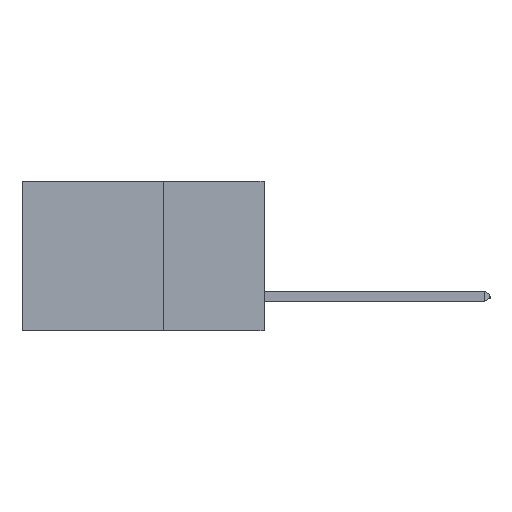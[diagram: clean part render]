
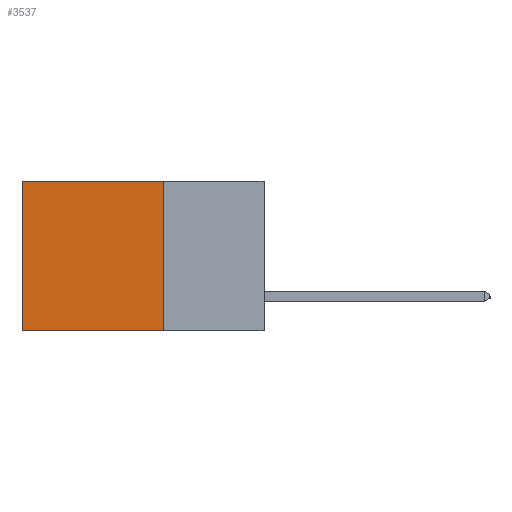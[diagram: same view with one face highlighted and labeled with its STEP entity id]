
A CAD part, left-side view. The second image highlights one B-rep face of the part: STEP entity #3537.
In plain terms, the highlighted planar face has unit normal (-1, 0, 0).
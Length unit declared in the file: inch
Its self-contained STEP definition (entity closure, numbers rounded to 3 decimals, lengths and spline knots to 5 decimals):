
#515 = VECTOR ( 'NONE', #7679, 39.37008 ) ;
#1892 = FACE_OUTER_BOUND ( 'NONE', #7209, .T. ) ;
#2263 = ORIENTED_EDGE ( 'NONE', *, *, #4184, .T. ) ;
#2540 = CARTESIAN_POINT ( 'NONE',  ( 0.298, 0.25, -0.37 ) ) ;
#2552 = CARTESIAN_POINT ( 'NONE',  ( 0.298, 0.25, -0.37 ) ) ;
#2980 = DIRECTION ( 'NONE',  ( 1., 0., 0. ) ) ;
#3294 = DIRECTION ( 'NONE',  ( 0., 0., -1. ) ) ;
#3537 = ADVANCED_FACE ( 'NONE', ( #1892 ), #13836, .F. ) ;
#3599 = VERTEX_POINT ( 'NONE', #7560 ) ;
#3607 = VECTOR ( 'NONE', #5527, 39.37008 ) ;
#4184 = EDGE_CURVE ( 'NONE', #3599, #9259, #11468, .T. ) ;
#4419 = LINE ( 'NONE', #2552, #515 ) ;
#4475 = ORIENTED_EDGE ( 'NONE', *, *, #8166, .F. ) ;
#5527 = DIRECTION ( 'NONE',  ( 0., 1., 0. ) ) ;
#7209 = EDGE_LOOP ( 'NONE', ( #2263, #10523, #4475, #12527 ) ) ;
#7462 = VECTOR ( 'NONE', #10243, 39.37008 ) ;
#7560 = CARTESIAN_POINT ( 'NONE',  ( 0.298, 0.6, 0. ) ) ;
#7679 = DIRECTION ( 'NONE',  ( 0., 1., 0. ) ) ;
#8166 = EDGE_CURVE ( 'NONE', #9520, #8747, #14227, .T. ) ;
#8747 = VERTEX_POINT ( 'NONE', #2540 ) ;
#8990 = CARTESIAN_POINT ( 'NONE',  ( 0.298, 0.25, 0. ) ) ;
#9180 = CARTESIAN_POINT ( 'NONE',  ( 0.298, 0.25, 0. ) ) ;
#9259 = VERTEX_POINT ( 'NONE', #11651 ) ;
#9520 = VERTEX_POINT ( 'NONE', #13674 ) ;
#10243 = DIRECTION ( 'NONE',  ( 0., 0., -1. ) ) ;
#10523 = ORIENTED_EDGE ( 'NONE', *, *, #10824, .F. ) ;
#10824 = EDGE_CURVE ( 'NONE', #8747, #9259, #4419, .T. ) ;
#11036 = VECTOR ( 'NONE', #15401, 39.37008 ) ;
#11468 = LINE ( 'NONE', #15200, #11036 ) ;
#11651 = CARTESIAN_POINT ( 'NONE',  ( 0.298, 0.6, -0.37 ) ) ;
#11734 = EDGE_CURVE ( 'NONE', #9520, #3599, #13756, .T. ) ;
#12527 = ORIENTED_EDGE ( 'NONE', *, *, #11734, .T. ) ;
#13169 = CARTESIAN_POINT ( 'NONE',  ( 0.298, 0.25, 0. ) ) ;
#13674 = CARTESIAN_POINT ( 'NONE',  ( 0.298, 0.25, 0. ) ) ;
#13756 = LINE ( 'NONE', #13169, #3607 ) ;
#13836 = PLANE ( 'NONE',  #15066 ) ;
#14227 = LINE ( 'NONE', #8990, #7462 ) ;
#15066 = AXIS2_PLACEMENT_3D ( 'NONE', #9180, #2980, #3294 ) ;
#15200 = CARTESIAN_POINT ( 'NONE',  ( 0.298, 0.6, 0. ) ) ;
#15401 = DIRECTION ( 'NONE',  ( 0., 0., -1. ) ) ;
